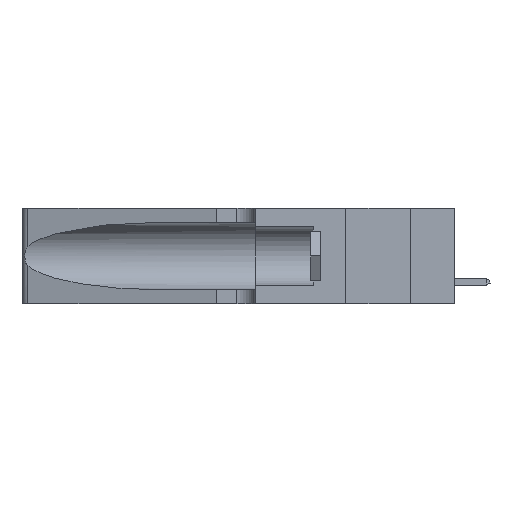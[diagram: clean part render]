
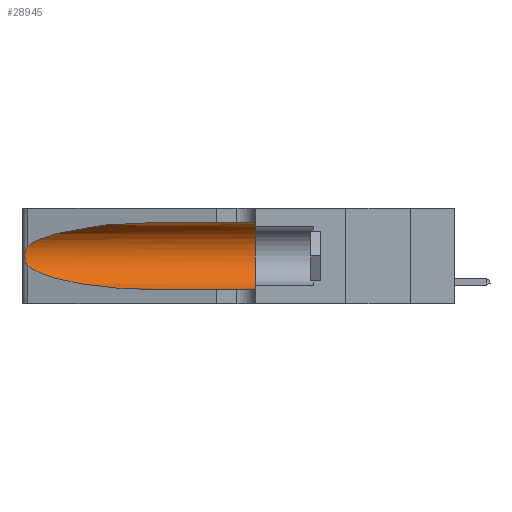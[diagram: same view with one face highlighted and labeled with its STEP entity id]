
A CAD part, left-side view. The second image highlights one B-rep face of the part: STEP entity #28945.
In plain terms, the highlighted cylindrical face has radius 3.308 mm (diameter 6.617 mm), a partial arc.
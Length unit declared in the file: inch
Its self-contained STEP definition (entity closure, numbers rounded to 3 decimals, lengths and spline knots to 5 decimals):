
#302 = CARTESIAN_POINT ( 'NONE',  ( 0.25639, 1.23186, 0.15144 ) ) ;
#1019 = CIRCLE ( 'NONE', #14786, 0.13025 ) ;
#1250 = ORIENTED_EDGE ( 'NONE', *, *, #48565, .T. ) ;
#4102 = CARTESIAN_POINT ( 'NONE',  ( 0.25487, 1.22718, 0.22369 ) ) ;
#4116 = CARTESIAN_POINT ( 'NONE',  ( 0.26075, 1.23896, 0.178 ) ) ;
#4285 = ORIENTED_EDGE ( 'NONE', *, *, #41632, .F. ) ;
#4416 = CARTESIAN_POINT ( 'NONE',  ( 0.25487, 1.22718, 0.22369 ) ) ;
#5503 = EDGE_CURVE ( 'NONE', #50578, #23027, #13752, .T. ) ;
#6300 = CARTESIAN_POINT ( 'NONE',  ( 0.1305, 1.61858, 0.31525 ) ) ;
#7746 = LINE ( 'NONE', #50198, #41315 ) ;
#8173 = CARTESIAN_POINT ( 'NONE',  ( 0.25639, 1.23184, 0.21858 ) ) ;
#8316 = CARTESIAN_POINT ( 'NONE',  ( 0.25487, 1.22718, 0.14631 ) ) ;
#8457 = CARTESIAN_POINT ( 'NONE',  ( 0.25854, 1.2359, 0.20912 ) ) ;
#11893 = CARTESIAN_POINT ( 'NONE',  ( 0.26018, 1.23835, 0.19895 ) ) ;
#13127 = LINE ( 'NONE', #6300, #32136 ) ;
#13403 = CARTESIAN_POINT ( 'NONE',  ( 0.18966, 0.96281, 0.31525 ) ) ;
#13752 =( BOUNDED_CURVE ( )  B_SPLINE_CURVE ( 3, ( #34914, #39123, #18996, #42761 ),
 .UNSPECIFIED., .F., .T. ) 
 B_SPLINE_CURVE_WITH_KNOTS ( ( 4, 4 ),
 ( 3.44316, 4.71239 ),
 .UNSPECIFIED. ) 
 CURVE ( )  GEOMETRIC_REPRESENTATION_ITEM ( )  RATIONAL_B_SPLINE_CURVE ( ( 1., 0.87, 0.87, 1. ) ) 
 REPRESENTATION_ITEM ( '' )  );
#14786 = AXIS2_PLACEMENT_3D ( 'NONE', #24940, #17251, #44595 ) ;
#15132 = DIRECTION ( 'NONE',  ( 0., -1., 0. ) ) ;
#16996 = CARTESIAN_POINT ( 'NONE',  ( 0.2373, 1.15595, 0.28018 ) ) ;
#17251 = DIRECTION ( 'NONE',  ( 0., 1., 0. ) ) ;
#18996 = CARTESIAN_POINT ( 'NONE',  ( 0.18966, 0.96281, 0.05475 ) ) ;
#19409 = CARTESIAN_POINT ( 'NONE',  ( 0.1305, 0.35, 0.05475 ) ) ;
#19863 = CARTESIAN_POINT ( 'NONE',  ( 0.1305, 0.72297, 0.31525 ) ) ;
#19875 = CARTESIAN_POINT ( 'NONE',  ( 0.26075, 1.23896, 0.19203 ) ) ;
#20193 = CARTESIAN_POINT ( 'NONE',  ( 0.25555, 1.22993, 0.14849 ) ) ;
#22149 = CARTESIAN_POINT ( 'NONE',  ( 0.25487, 1.22718, 0.14631 ) ) ;
#22318 = CARTESIAN_POINT ( 'NONE',  ( 0.1305, 0.35, 0.31525 ) ) ;
#23027 = VERTEX_POINT ( 'NONE', #41157 ) ;
#23368 = DIRECTION ( 'NONE',  ( 0., 0., -1. ) ) ;
#24940 = CARTESIAN_POINT ( 'NONE',  ( 0.1305, 0.35, 0.185 ) ) ;
#26101 = EDGE_CURVE ( 'NONE', #37960, #47151, #1019, .T. ) ;
#26687 = FACE_OUTER_BOUND ( 'NONE', #32646, .T. ) ;
#26702 =( BOUNDED_CURVE ( )  B_SPLINE_CURVE ( 3, ( #48603, #13403, #16996, #40734 ),
 .UNSPECIFIED., .F., .F. ) 
 B_SPLINE_CURVE_WITH_KNOTS ( ( 4, 4 ),
 ( 1.5708, 2.84003 ),
 .UNSPECIFIED. ) 
 CURVE ( )  GEOMETRIC_REPRESENTATION_ITEM ( )  RATIONAL_B_SPLINE_CURVE ( ( 1., 0.87, 0.87, 1. ) ) 
 REPRESENTATION_ITEM ( '' )  );
#28945 = ADVANCED_FACE ( 'NONE', ( #26687 ), #32048, .F. ) ;
#29417 = ORIENTED_EDGE ( 'NONE', *, *, #41324, .T. ) ;
#31326 = B_SPLINE_CURVE_WITH_KNOTS ( 'NONE', 3,
 ( #4416, #43312, #8173, #31696, #8457, #11893, #19875, #4116, #43620, #47269, #35619, #302, #20193, #8316 ),
 .UNSPECIFIED., .F., .F.,
 ( 4, 2, 2, 2, 2, 2, 4 ),
 ( 0., 0.00027, 0.00053, 0.00107, 0.0016, 0.00187, 0.00214 ),
 .UNSPECIFIED. ) ;
#31696 = CARTESIAN_POINT ( 'NONE',  ( 0.25787, 1.23484, 0.2124 ) ) ;
#32048 = CYLINDRICAL_SURFACE ( 'NONE', #44567, 0.13025 ) ;
#32136 = VECTOR ( 'NONE', #33398, 39.37008 ) ;
#32646 = EDGE_LOOP ( 'NONE', ( #1250, #29417, #47020, #39692, #46810, #4285 ) ) ;
#33398 = DIRECTION ( 'NONE',  ( 0., -1., 0. ) ) ;
#34914 = CARTESIAN_POINT ( 'NONE',  ( 0.25487, 1.22718, 0.14631 ) ) ;
#35619 = CARTESIAN_POINT ( 'NONE',  ( 0.25789, 1.23486, 0.15765 ) ) ;
#37960 = VERTEX_POINT ( 'NONE', #22318 ) ;
#39123 = CARTESIAN_POINT ( 'NONE',  ( 0.2373, 1.15595, 0.08982 ) ) ;
#39692 = ORIENTED_EDGE ( 'NONE', *, *, #41810, .T. ) ;
#40734 = CARTESIAN_POINT ( 'NONE',  ( 0.25487, 1.22718, 0.22369 ) ) ;
#41157 = CARTESIAN_POINT ( 'NONE',  ( 0.1305, 0.72297, 0.05475 ) ) ;
#41315 = VECTOR ( 'NONE', #15132, 39.37008 ) ;
#41324 = EDGE_CURVE ( 'NONE', #43270, #50578, #31326, .T. ) ;
#41632 = EDGE_CURVE ( 'NONE', #45452, #37960, #13127, .T. ) ;
#41810 = EDGE_CURVE ( 'NONE', #23027, #47151, #7746, .T. ) ;
#42761 = CARTESIAN_POINT ( 'NONE',  ( 0.1305, 0.72297, 0.05475 ) ) ;
#43270 = VERTEX_POINT ( 'NONE', #4102 ) ;
#43312 = CARTESIAN_POINT ( 'NONE',  ( 0.25555, 1.22994, 0.2215 ) ) ;
#43620 = CARTESIAN_POINT ( 'NONE',  ( 0.26017, 1.23833, 0.17102 ) ) ;
#44567 = AXIS2_PLACEMENT_3D ( 'NONE', #47068, #50539, #23368 ) ;
#44595 = DIRECTION ( 'NONE',  ( 0., 0., 1. ) ) ;
#45452 = VERTEX_POINT ( 'NONE', #19863 ) ;
#46810 = ORIENTED_EDGE ( 'NONE', *, *, #26101, .F. ) ;
#47020 = ORIENTED_EDGE ( 'NONE', *, *, #5503, .T. ) ;
#47068 = CARTESIAN_POINT ( 'NONE',  ( 0.1305, 1.61858, 0.185 ) ) ;
#47151 = VERTEX_POINT ( 'NONE', #19409 ) ;
#47269 = CARTESIAN_POINT ( 'NONE',  ( 0.25856, 1.23593, 0.16098 ) ) ;
#48565 = EDGE_CURVE ( 'NONE', #45452, #43270, #26702, .T. ) ;
#48603 = CARTESIAN_POINT ( 'NONE',  ( 0.1305, 0.72297, 0.31525 ) ) ;
#50198 = CARTESIAN_POINT ( 'NONE',  ( 0.1305, 1.61858, 0.05475 ) ) ;
#50539 = DIRECTION ( 'NONE',  ( 0., -1., 0. ) ) ;
#50578 = VERTEX_POINT ( 'NONE', #22149 ) ;
